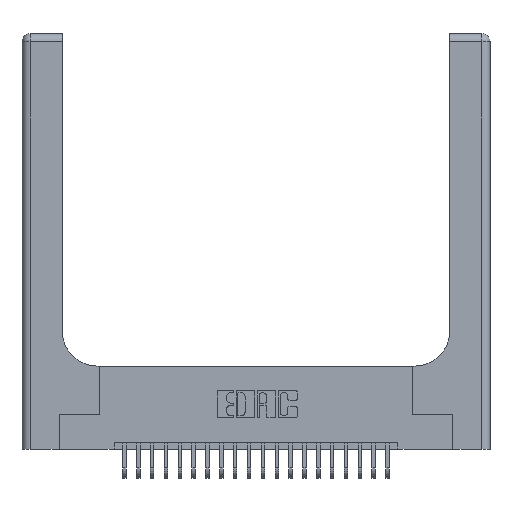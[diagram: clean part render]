
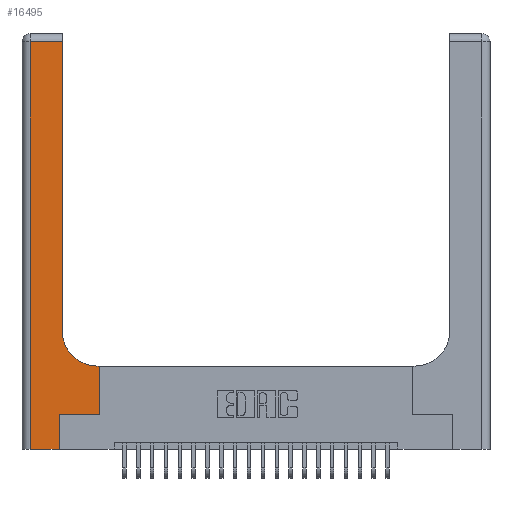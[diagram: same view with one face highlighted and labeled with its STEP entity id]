
A CAD part, top view. The second image highlights one B-rep face of the part: STEP entity #16495.
In plain terms, the highlighted planar face has unit normal (0, 0, 1).
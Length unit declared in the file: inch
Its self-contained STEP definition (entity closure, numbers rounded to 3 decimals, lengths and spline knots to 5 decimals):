
#520 = DIRECTION ( 'NONE',  ( 0., 1., 0. ) ) ;
#871 = CARTESIAN_POINT ( 'NONE',  ( 0.2915, 3., 0.37 ) ) ;
#1410 = CARTESIAN_POINT ( 'NONE',  ( 0., 0., 0.37 ) ) ;
#1584 = VERTEX_POINT ( 'NONE', #10382 ) ;
#2427 = VERTEX_POINT ( 'NONE', #5195 ) ;
#2434 = EDGE_CURVE ( 'NONE', #24676, #1584, #4085, .T. ) ;
#2530 = VECTOR ( 'NONE', #10954, 39.37008 ) ;
#2732 = EDGE_CURVE ( 'NONE', #3329, #24676, #23747, .T. ) ;
#2796 = CARTESIAN_POINT ( 'NONE',  ( 0.2915, 0.85, 0.37 ) ) ;
#3178 = LINE ( 'NONE', #871, #2530 ) ;
#3329 = VERTEX_POINT ( 'NONE', #10131 ) ;
#4085 = LINE ( 'NONE', #15147, #24309 ) ;
#4813 = CARTESIAN_POINT ( 'NONE',  ( 0., 3., 0.37 ) ) ;
#5195 = CARTESIAN_POINT ( 'NONE',  ( 0.2915, 2.94, 0.37 ) ) ;
#6053 = EDGE_CURVE ( 'NONE', #20118, #16938, #10577, .T. ) ;
#6868 = EDGE_LOOP ( 'NONE', ( #13989, #19158, #24800, #15225, #20948, #16441, #17648, #23323, #13699 ) ) ;
#7492 = DIRECTION ( 'NONE',  ( 1., 0., 0. ) ) ;
#8045 = VECTOR ( 'NONE', #7492, 39.37008 ) ;
#8213 = VECTOR ( 'NONE', #15983, 39.37008 ) ;
#8896 = DIRECTION ( 'NONE',  ( -1., 0., 0. ) ) ;
#9497 = CARTESIAN_POINT ( 'NONE',  ( 0., 2.94, 0.37 ) ) ;
#9731 = VECTOR ( 'NONE', #520, 39.37008 ) ;
#10131 = CARTESIAN_POINT ( 'NONE',  ( 0.269, 0., 0.37 ) ) ;
#10276 = CARTESIAN_POINT ( 'NONE',  ( 0.5415, 0.85, 0.37 ) ) ;
#10382 = CARTESIAN_POINT ( 'NONE',  ( 0.5585, 0.25, 0.37 ) ) ;
#10577 = CIRCLE ( 'NONE', #17226, 0.25 ) ;
#10648 = EDGE_CURVE ( 'NONE', #19873, #20297, #19519, .T. ) ;
#10876 = DIRECTION ( 'NONE',  ( 0., -1., 0. ) ) ;
#10954 = DIRECTION ( 'NONE',  ( 0., 1., 0. ) ) ;
#11046 = CARTESIAN_POINT ( 'NONE',  ( 0.06, 2.94, 0.37 ) ) ;
#11273 = DIRECTION ( 'NONE',  ( 1., 0., 0. ) ) ;
#11888 = CARTESIAN_POINT ( 'NONE',  ( 0.5415, 0.6, 0.37 ) ) ;
#11955 = EDGE_CURVE ( 'NONE', #2427, #19873, #20045, .T. ) ;
#12209 = CARTESIAN_POINT ( 'NONE',  ( 0.5585, 0.25, 0.37 ) ) ;
#12241 = DIRECTION ( 'NONE',  ( 1., 0., 0. ) ) ;
#12303 = VECTOR ( 'NONE', #24129, 39.37008 ) ;
#13341 = LINE ( 'NONE', #1410, #8045 ) ;
#13699 = ORIENTED_EDGE ( 'NONE', *, *, #6053, .T. ) ;
#13750 = VECTOR ( 'NONE', #10876, 39.37008 ) ;
#13989 = ORIENTED_EDGE ( 'NONE', *, *, #25207, .T. ) ;
#14970 = LINE ( 'NONE', #12209, #9731 ) ;
#15147 = CARTESIAN_POINT ( 'NONE',  ( 0.269, 0.25, 0.37 ) ) ;
#15225 = ORIENTED_EDGE ( 'NONE', *, *, #22506, .T. ) ;
#15351 = CARTESIAN_POINT ( 'NONE',  ( 0.269, 0.25, 0.37 ) ) ;
#15983 = DIRECTION ( 'NONE',  ( 0., 1., 0. ) ) ;
#16250 = AXIS2_PLACEMENT_3D ( 'NONE', #4813, #20594, #8896 ) ;
#16441 = ORIENTED_EDGE ( 'NONE', *, *, #2434, .T. ) ;
#16495 = ADVANCED_FACE ( 'NONE', ( #17763 ), #18684, .F. ) ;
#16938 = VERTEX_POINT ( 'NONE', #2796 ) ;
#17226 = AXIS2_PLACEMENT_3D ( 'NONE', #10276, #23797, #12241 ) ;
#17487 = LINE ( 'NONE', #20306, #12303 ) ;
#17648 = ORIENTED_EDGE ( 'NONE', *, *, #17871, .T. ) ;
#17763 = FACE_OUTER_BOUND ( 'NONE', #6868, .T. ) ;
#17871 = EDGE_CURVE ( 'NONE', #1584, #18930, #14970, .T. ) ;
#18684 = PLANE ( 'NONE',  #16250 ) ;
#18930 = VERTEX_POINT ( 'NONE', #25251 ) ;
#19158 = ORIENTED_EDGE ( 'NONE', *, *, #11955, .T. ) ;
#19519 = LINE ( 'NONE', #22547, #13750 ) ;
#19873 = VERTEX_POINT ( 'NONE', #11046 ) ;
#20045 = LINE ( 'NONE', #9497, #25104 ) ;
#20118 = VERTEX_POINT ( 'NONE', #11888 ) ;
#20297 = VERTEX_POINT ( 'NONE', #22110 ) ;
#20306 = CARTESIAN_POINT ( 'NONE',  ( 0.2915, 0.6, 0.37 ) ) ;
#20594 = DIRECTION ( 'NONE',  ( 0., 0., -1. ) ) ;
#20948 = ORIENTED_EDGE ( 'NONE', *, *, #2732, .T. ) ;
#21152 = DIRECTION ( 'NONE',  ( -1., 0., 0. ) ) ;
#22110 = CARTESIAN_POINT ( 'NONE',  ( 0.06, 0., 0.37 ) ) ;
#22197 = EDGE_CURVE ( 'NONE', #18930, #20118, #17487, .T. ) ;
#22506 = EDGE_CURVE ( 'NONE', #20297, #3329, #13341, .T. ) ;
#22547 = CARTESIAN_POINT ( 'NONE',  ( 0.06, 3., 0.37 ) ) ;
#23323 = ORIENTED_EDGE ( 'NONE', *, *, #22197, .T. ) ;
#23747 = LINE ( 'NONE', #25524, #8213 ) ;
#23797 = DIRECTION ( 'NONE',  ( 0., 0., -1. ) ) ;
#24129 = DIRECTION ( 'NONE',  ( -1., 0., 0. ) ) ;
#24309 = VECTOR ( 'NONE', #11273, 39.37008 ) ;
#24676 = VERTEX_POINT ( 'NONE', #15351 ) ;
#24800 = ORIENTED_EDGE ( 'NONE', *, *, #10648, .T. ) ;
#25104 = VECTOR ( 'NONE', #21152, 39.37008 ) ;
#25207 = EDGE_CURVE ( 'NONE', #16938, #2427, #3178, .T. ) ;
#25251 = CARTESIAN_POINT ( 'NONE',  ( 0.5585, 0.6, 0.37 ) ) ;
#25524 = CARTESIAN_POINT ( 'NONE',  ( 0.269, 0., 0.37 ) ) ;
